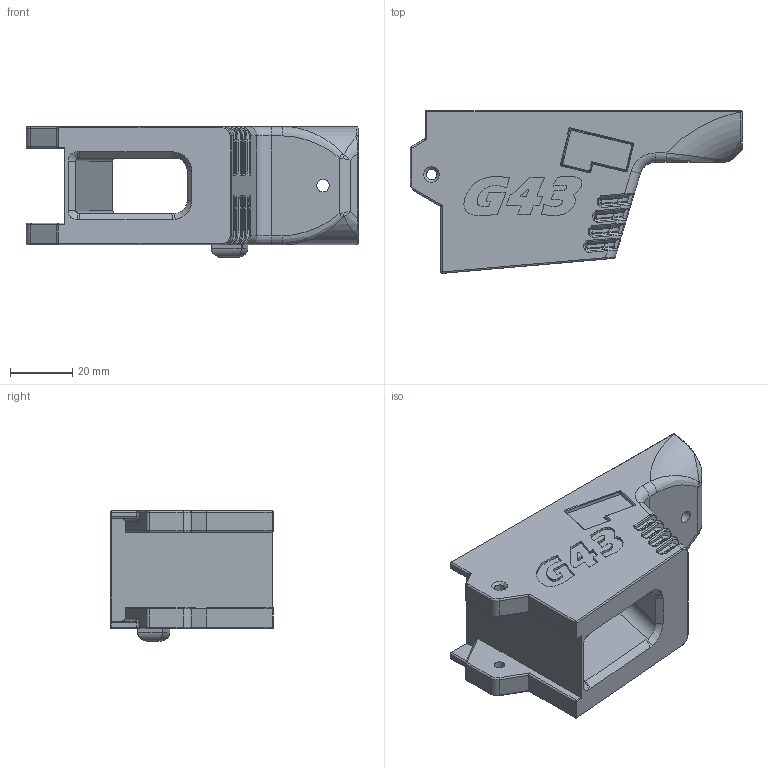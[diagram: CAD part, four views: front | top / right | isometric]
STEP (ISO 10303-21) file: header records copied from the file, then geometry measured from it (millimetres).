
FILE_DESCRIPTION(/* description */ (''),/* implementation_level */ '2;1');
FILE_NAME(/* name */ 'MOD9 G43 Magwell.stp',/* time_stamp */ '2020-10-20T11:55:13+03:00',/* author */ (''),/* organization */ (''),/* preprocessor_version */ 'ST-DEVELOPER v15.2',/* originating_system */ 'Autodesk Translator Framework v2.0.0.5431',/* authorisation */ '');
FILE_SCHEMA (('AUTOMOTIVE_DESIGN { 1 0 10303 214 3 1 1 }'));
Length unit declared in the file: centimetre
Products named in the file (1): MOD9 G43v2
Bounding box: 106.51 x 52.16 x 42 mm (x, y, z)
Volume: 98085.1 mm3; surface area: 27393.3 mm2
Topology: 2 solids, 2 shells, 1000 faces, 2578 edges, 1577 vertices
Faces by surface type: bspline 434, cylinder 263, plane 252, sphere 20, cone 18, torus 13
Full cylindrical faces by diameter (mm): 1.5 x2, 3.4 x2, 4 x2
Entity records: 37573 total; most frequent: CARTESIAN_POINT 15818, ORIENTED_EDGE 5110, DIRECTION 3537, EDGE_CURVE 2555, VERTEX_POINT 1576, AXIS2_PLACEMENT_3D 1208, LINE 1121, VECTOR 1121
